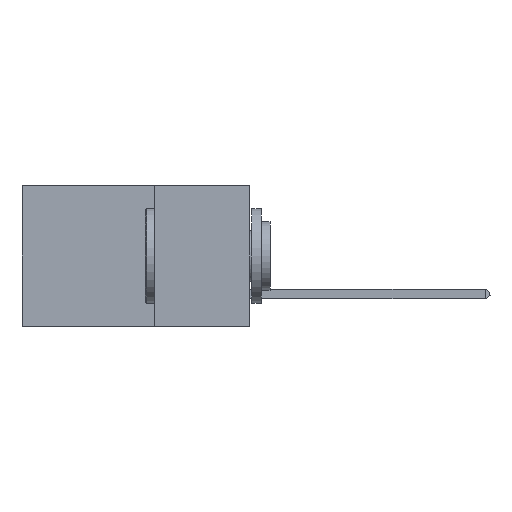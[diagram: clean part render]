
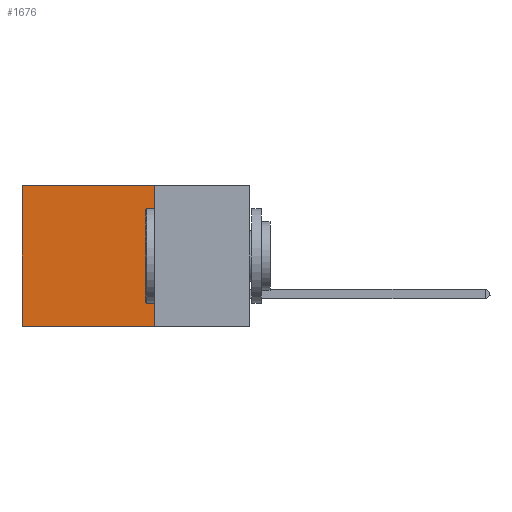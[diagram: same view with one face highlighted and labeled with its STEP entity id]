
A CAD part, left-side view. The second image highlights one B-rep face of the part: STEP entity #1676.
In plain terms, the highlighted planar face has unit normal (-1, 0, 0).
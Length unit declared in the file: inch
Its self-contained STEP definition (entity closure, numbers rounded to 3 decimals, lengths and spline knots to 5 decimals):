
#1185 = DIRECTION ( 'NONE',  ( 0., 0., -1. ) ) ;
#1676 = ADVANCED_FACE ( 'NONE', ( #42820 ), #3465, .F. ) ;
#3465 = PLANE ( 'NONE',  #3846 ) ;
#3846 = AXIS2_PLACEMENT_3D ( 'NONE', #15129, #22844, #14807 ) ;
#4237 = VERTEX_POINT ( 'NONE', #46013 ) ;
#5564 = VECTOR ( 'NONE', #1185, 39.37008 ) ;
#6404 = VERTEX_POINT ( 'NONE', #41396 ) ;
#6718 = VECTOR ( 'NONE', #42913, 39.37008 ) ;
#11001 = VECTOR ( 'NONE', #11122, 39.37008 ) ;
#11122 = DIRECTION ( 'NONE',  ( 0., 0., -1. ) ) ;
#13981 = VECTOR ( 'NONE', #36180, 39.37008 ) ;
#14807 = DIRECTION ( 'NONE',  ( 0., 0., -1. ) ) ;
#15129 = CARTESIAN_POINT ( 'NONE',  ( 0.2875, 0.25, 0. ) ) ;
#16713 = LINE ( 'NONE', #27473, #6718 ) ;
#18106 = ORIENTED_EDGE ( 'NONE', *, *, #23563, .T. ) ;
#19992 = EDGE_LOOP ( 'NONE', ( #18106, #40455, #24886, #29164 ) ) ;
#22528 = CARTESIAN_POINT ( 'NONE',  ( 0.2875, 0.25, -0.37 ) ) ;
#22844 = DIRECTION ( 'NONE',  ( 1., 0., 0. ) ) ;
#23563 = EDGE_CURVE ( 'NONE', #4237, #6404, #36738, .T. ) ;
#24886 = ORIENTED_EDGE ( 'NONE', *, *, #42527, .F. ) ;
#25710 = LINE ( 'NONE', #39737, #13981 ) ;
#27435 = CARTESIAN_POINT ( 'NONE',  ( 0.2875, 0.25, 0. ) ) ;
#27473 = CARTESIAN_POINT ( 'NONE',  ( 0.2875, 0.25, -0.37 ) ) ;
#28242 = EDGE_CURVE ( 'NONE', #41091, #4237, #25710, .T. ) ;
#29164 = ORIENTED_EDGE ( 'NONE', *, *, #28242, .T. ) ;
#30026 = CARTESIAN_POINT ( 'NONE',  ( 0.2875, 0.25, 0. ) ) ;
#36180 = DIRECTION ( 'NONE',  ( 0., 1., 0. ) ) ;
#36738 = LINE ( 'NONE', #40374, #11001 ) ;
#37296 = VERTEX_POINT ( 'NONE', #22528 ) ;
#39737 = CARTESIAN_POINT ( 'NONE',  ( 0.2875, 0.25, 0. ) ) ;
#40374 = CARTESIAN_POINT ( 'NONE',  ( 0.2875, 0.6, 0. ) ) ;
#40455 = ORIENTED_EDGE ( 'NONE', *, *, #42901, .F. ) ;
#41091 = VERTEX_POINT ( 'NONE', #30026 ) ;
#41396 = CARTESIAN_POINT ( 'NONE',  ( 0.2875, 0.6, -0.37 ) ) ;
#42527 = EDGE_CURVE ( 'NONE', #41091, #37296, #48250, .T. ) ;
#42820 = FACE_OUTER_BOUND ( 'NONE', #19992, .T. ) ;
#42901 = EDGE_CURVE ( 'NONE', #37296, #6404, #16713, .T. ) ;
#42913 = DIRECTION ( 'NONE',  ( 0., 1., 0. ) ) ;
#46013 = CARTESIAN_POINT ( 'NONE',  ( 0.2875, 0.6, 0. ) ) ;
#48250 = LINE ( 'NONE', #27435, #5564 ) ;
